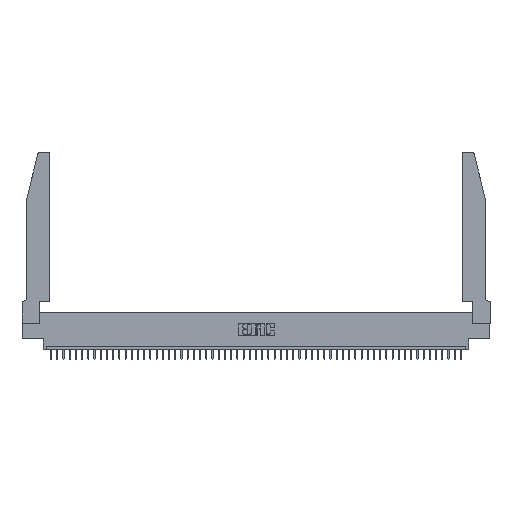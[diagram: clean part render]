
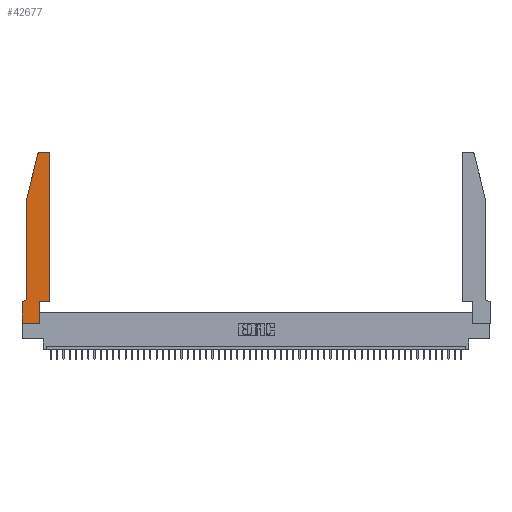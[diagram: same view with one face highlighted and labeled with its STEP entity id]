
A CAD part, top view. The second image highlights one B-rep face of the part: STEP entity #42677.
In plain terms, the highlighted planar face has unit normal (0, 0, 1).
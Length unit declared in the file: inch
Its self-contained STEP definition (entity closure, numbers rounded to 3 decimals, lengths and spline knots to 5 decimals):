
#113 = EDGE_CURVE ( 'NONE', #9876, #26081, #23863, .T. ) ;
#163 = AXIS2_PLACEMENT_3D ( 'NONE', #6599, #38302, #46649 ) ;
#828 = VERTEX_POINT ( 'NONE', #5818 ) ;
#1852 = VECTOR ( 'NONE', #21034, 39.37008 ) ;
#1977 = EDGE_CURVE ( 'NONE', #45271, #9876, #6675, .T. ) ;
#2563 = VERTEX_POINT ( 'NONE', #33257 ) ;
#2762 = ORIENTED_EDGE ( 'NONE', *, *, #113, .T. ) ;
#2805 = DIRECTION ( 'NONE',  ( -1., 0., 0. ) ) ;
#3434 = VECTOR ( 'NONE', #2805, 39.37008 ) ;
#4625 = CARTESIAN_POINT ( 'NONE',  ( 0.4505, 0.35, 0.37 ) ) ;
#5818 = CARTESIAN_POINT ( 'NONE',  ( 0.4505, 2.72, 0.37 ) ) ;
#6394 = LINE ( 'NONE', #28762, #13875 ) ;
#6599 = CARTESIAN_POINT ( 'NONE',  ( 0., 0.35, 0.37 ) ) ;
#6675 = LINE ( 'NONE', #34802, #41753 ) ;
#6822 = DIRECTION ( 'NONE',  ( 1., 0., 0. ) ) ;
#7602 = ORIENTED_EDGE ( 'NONE', *, *, #27332, .T. ) ;
#7927 = VECTOR ( 'NONE', #8924, 39.37008 ) ;
#8003 = EDGE_CURVE ( 'NONE', #828, #38348, #35827, .T. ) ;
#8924 = DIRECTION ( 'NONE',  ( -1., 0., 0. ) ) ;
#9501 = ORIENTED_EDGE ( 'NONE', *, *, #49249, .T. ) ;
#9656 = CARTESIAN_POINT ( 'NONE',  ( 0.0755, 2., 0.37 ) ) ;
#9759 = CARTESIAN_POINT ( 'NONE',  ( 0.4505, 0.35, 0.37 ) ) ;
#9876 = VERTEX_POINT ( 'NONE', #9656 ) ;
#9975 = VERTEX_POINT ( 'NONE', #19443 ) ;
#10834 = DIRECTION ( 'NONE',  ( 0., 1., 0. ) ) ;
#12114 = CARTESIAN_POINT ( 'NONE',  ( 0.2605, 2.75, 0.37 ) ) ;
#12196 = VECTOR ( 'NONE', #10834, 39.37008 ) ;
#13168 = VERTEX_POINT ( 'NONE', #36402 ) ;
#13875 = VECTOR ( 'NONE', #14054, 39.37008 ) ;
#14054 = DIRECTION ( 'NONE',  ( 0., -1., 0. ) ) ;
#14458 = DIRECTION ( 'NONE',  ( 0., 0., 1. ) ) ;
#14766 = ORIENTED_EDGE ( 'NONE', *, *, #28056, .T. ) ;
#17035 = ORIENTED_EDGE ( 'NONE', *, *, #27396, .T. ) ;
#18253 = EDGE_LOOP ( 'NONE', ( #17035, #9501, #41432, #2762, #38077, #44236, #46333, #32402, #42023, #7602, #14766, #44684 ) ) ;
#18611 = CARTESIAN_POINT ( 'NONE',  ( 0.4505, 0.35, 0.37 ) ) ;
#18799 = DIRECTION ( 'NONE',  ( 1., 0., 0. ) ) ;
#19415 = DIRECTION ( 'NONE',  ( 0., 0., -1. ) ) ;
#19443 = CARTESIAN_POINT ( 'NONE',  ( 0.0055, 0.35, 0.37 ) ) ;
#21034 = DIRECTION ( 'NONE',  ( 0., -1., 0. ) ) ;
#22124 = PLANE ( 'NONE',  #163 ) ;
#22516 = VERTEX_POINT ( 'NONE', #4625 ) ;
#22817 = LINE ( 'NONE', #34413, #12196 ) ;
#23863 = LINE ( 'NONE', #26474, #1852 ) ;
#24712 = VERTEX_POINT ( 'NONE', #44609 ) ;
#25384 = CARTESIAN_POINT ( 'NONE',  ( 0., 0., 0.37 ) ) ;
#25455 = AXIS2_PLACEMENT_3D ( 'NONE', #26659, #19415, #43568 ) ;
#25907 = VECTOR ( 'NONE', #30221, 39.37008 ) ;
#26081 = VERTEX_POINT ( 'NONE', #33427 ) ;
#26195 = EDGE_CURVE ( 'NONE', #9975, #27753, #39270, .T. ) ;
#26474 = CARTESIAN_POINT ( 'NONE',  ( 0.0755, 2., 0.37 ) ) ;
#26659 = CARTESIAN_POINT ( 'NONE',  ( 0.0055, 0.42, 0.37 ) ) ;
#26687 = FACE_OUTER_BOUND ( 'NONE', #18253, .T. ) ;
#26965 = DIRECTION ( 'NONE',  ( 1., 0., 0. ) ) ;
#27260 = AXIS2_PLACEMENT_3D ( 'NONE', #30771, #14458, #51793 ) ;
#27315 = EDGE_CURVE ( 'NONE', #2563, #24712, #22817, .T. ) ;
#27332 = EDGE_CURVE ( 'NONE', #24712, #22516, #50497, .T. ) ;
#27396 = EDGE_CURVE ( 'NONE', #38348, #50283, #30285, .T. ) ;
#27753 = VERTEX_POINT ( 'NONE', #49670 ) ;
#28056 = EDGE_CURVE ( 'NONE', #22516, #828, #47421, .T. ) ;
#28762 = CARTESIAN_POINT ( 'NONE',  ( 0., 0., 0.37 ) ) ;
#30221 = DIRECTION ( 'NONE',  ( 0., 1., 0. ) ) ;
#30285 = LINE ( 'NONE', #12114, #3434 ) ;
#30771 = CARTESIAN_POINT ( 'NONE',  ( 0.4205, 2.72, 0.37 ) ) ;
#31169 = EDGE_CURVE ( 'NONE', #13168, #2563, #43930, .T. ) ;
#31761 = CARTESIAN_POINT ( 'NONE',  ( 0.25487, 2.72718, 0.37 ) ) ;
#32402 = ORIENTED_EDGE ( 'NONE', *, *, #31169, .T. ) ;
#33188 = CARTESIAN_POINT ( 'NONE',  ( 0.4205, 2.75, 0.37 ) ) ;
#33257 = CARTESIAN_POINT ( 'NONE',  ( 0.2865, 0., 0.37 ) ) ;
#33427 = CARTESIAN_POINT ( 'NONE',  ( 0.0755, 0.42, 0.37 ) ) ;
#33702 = CIRCLE ( 'NONE', #25455, 0.07 ) ;
#34413 = CARTESIAN_POINT ( 'NONE',  ( 0.2865, 0.35, 0.37 ) ) ;
#34802 = CARTESIAN_POINT ( 'NONE',  ( 0.0755, 2., 0.37 ) ) ;
#35827 = CIRCLE ( 'NONE', #27260, 0.03 ) ;
#35883 = EDGE_CURVE ( 'NONE', #27753, #13168, #6394, .T. ) ;
#36402 = CARTESIAN_POINT ( 'NONE',  ( 0., 0., 0.37 ) ) ;
#36972 = CARTESIAN_POINT ( 'NONE',  ( 0.0755, 0.35, 0.37 ) ) ;
#37351 = CARTESIAN_POINT ( 'NONE',  ( 0.284, 2.75, 0.37 ) ) ;
#38077 = ORIENTED_EDGE ( 'NONE', *, *, #50520, .T. ) ;
#38302 = DIRECTION ( 'NONE',  ( 0., 0., 1. ) ) ;
#38348 = VERTEX_POINT ( 'NONE', #33188 ) ;
#39270 = LINE ( 'NONE', #36972, #7927 ) ;
#40400 = VECTOR ( 'NONE', #18799, 39.37008 ) ;
#40730 = VECTOR ( 'NONE', #26965, 39.37008 ) ;
#41432 = ORIENTED_EDGE ( 'NONE', *, *, #1977, .T. ) ;
#41753 = VECTOR ( 'NONE', #42937, 39.37008 ) ;
#42023 = ORIENTED_EDGE ( 'NONE', *, *, #27315, .T. ) ;
#42677 = ADVANCED_FACE ( 'NONE', ( #26687 ), #22124, .T. ) ;
#42937 = DIRECTION ( 'NONE',  ( -0.239, -0.971, 0. ) ) ;
#43568 = DIRECTION ( 'NONE',  ( -1., 0., 0. ) ) ;
#43930 = LINE ( 'NONE', #25384, #40730 ) ;
#44236 = ORIENTED_EDGE ( 'NONE', *, *, #26195, .T. ) ;
#44609 = CARTESIAN_POINT ( 'NONE',  ( 0.2865, 0.35, 0.37 ) ) ;
#44684 = ORIENTED_EDGE ( 'NONE', *, *, #8003, .T. ) ;
#45271 = VERTEX_POINT ( 'NONE', #31761 ) ;
#45674 = AXIS2_PLACEMENT_3D ( 'NONE', #51289, #47065, #6822 ) ;
#46333 = ORIENTED_EDGE ( 'NONE', *, *, #35883, .T. ) ;
#46649 = DIRECTION ( 'NONE',  ( 1., 0., 0. ) ) ;
#47065 = DIRECTION ( 'NONE',  ( 0., 0., 1. ) ) ;
#47421 = LINE ( 'NONE', #9759, #25907 ) ;
#48955 = CIRCLE ( 'NONE', #45674, 0.03 ) ;
#49249 = EDGE_CURVE ( 'NONE', #50283, #45271, #48955, .T. ) ;
#49670 = CARTESIAN_POINT ( 'NONE',  ( 0., 0.35, 0.37 ) ) ;
#50283 = VERTEX_POINT ( 'NONE', #37351 ) ;
#50497 = LINE ( 'NONE', #18611, #40400 ) ;
#50520 = EDGE_CURVE ( 'NONE', #26081, #9975, #33702, .T. ) ;
#51289 = CARTESIAN_POINT ( 'NONE',  ( 0.284, 2.72, 0.37 ) ) ;
#51793 = DIRECTION ( 'NONE',  ( 1., 0., 0. ) ) ;
